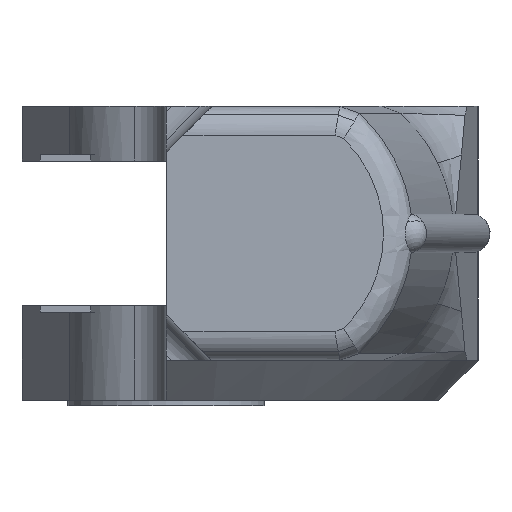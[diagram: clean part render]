
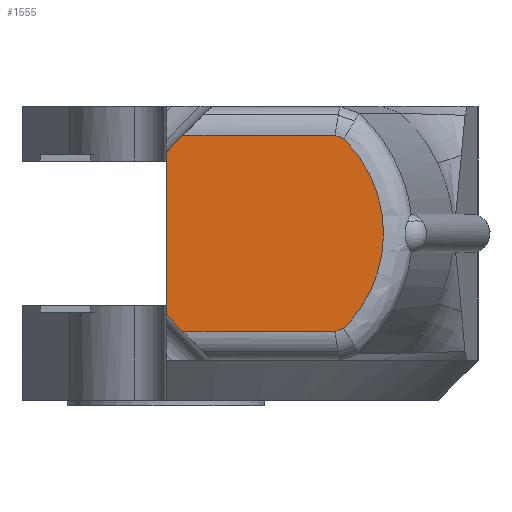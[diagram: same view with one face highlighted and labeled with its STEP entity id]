
A CAD part, left-side view. The second image highlights one B-rep face of the part: STEP entity #1555.
In plain terms, the highlighted planar face has unit normal (-1, 0, 0).
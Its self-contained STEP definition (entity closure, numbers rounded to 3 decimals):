
#22 = CARTESIAN_POINT ( 'NONE',  ( -27.856, 0., -2.85 ) ) ;
#83 = ORIENTED_EDGE ( 'NONE', *, *, #1610, .F. ) ;
#96 = DIRECTION ( 'NONE',  ( -1., 0., 0. ) ) ;
#164 = VECTOR ( 'NONE', #2389, 1000. ) ;
#197 = ORIENTED_EDGE ( 'NONE', *, *, #1725, .F. ) ;
#244 = VECTOR ( 'NONE', #807, 1000. ) ;
#266 = CARTESIAN_POINT ( 'NONE',  ( -27.856, -0.091, 2.941 ) ) ;
#279 = CARTESIAN_POINT ( 'NONE',  ( -27.856, 0., 0. ) ) ;
#336 = VECTOR ( 'NONE', #1314, 1000. ) ;
#350 = DIRECTION ( 'NONE',  ( 0., 1., 0. ) ) ;
#390 = DIRECTION ( 'NONE',  ( 0., -0.939, -0.343 ) ) ;
#400 = VERTEX_POINT ( 'NONE', #1498 ) ;
#481 = CARTESIAN_POINT ( 'NONE',  ( -27.856, 0., 2.85 ) ) ;
#652 = CARTESIAN_POINT ( 'NONE',  ( -27.856, -3.89, 4.185 ) ) ;
#695 = CARTESIAN_POINT ( 'NONE',  ( -27.856, -6.233, 3.329 ) ) ;
#807 = DIRECTION ( 'NONE',  ( 0., 0.707, -0.707 ) ) ;
#813 = VECTOR ( 'NONE', #350, 1000. ) ;
#892 = CARTESIAN_POINT ( 'NONE',  ( -27.856, -2.016, 3.442 ) ) ;
#923 = VECTOR ( 'NONE', #1765, 1000. ) ;
#926 = CARTESIAN_POINT ( 'NONE',  ( -27.856, -0.591, -3.442 ) ) ;
#934 = VERTEX_POINT ( 'NONE', #22 ) ;
#944 = LINE ( 'NONE', #279, #164 ) ;
#1031 = LINE ( 'NONE', #1042, #336 ) ;
#1038 = VERTEX_POINT ( 'NONE', #1669 ) ;
#1042 = CARTESIAN_POINT ( 'NONE',  ( -27.856, 0.713, -2.138 ) ) ;
#1099 = CARTESIAN_POINT ( 'NONE',  ( -27.856, -5.925, 3.442 ) ) ;
#1104 = VERTEX_POINT ( 'NONE', #1716 ) ;
#1221 = CARTESIAN_POINT ( 'NONE',  ( -27.856, -8.217, -1.386 ) ) ;
#1314 = DIRECTION ( 'NONE',  ( 0., -0.707, -0.707 ) ) ;
#1444 = EDGE_LOOP ( 'NONE', ( #3081, #197, #3039, #83, #2172, #3075, #2840, #2040 ) ) ;
#1498 = CARTESIAN_POINT ( 'NONE',  ( -27.856, -0.591, 3.442 ) ) ;
#1535 = EDGE_CURVE ( 'NONE', #1038, #1642, #2214, .T. ) ;
#1555 = ADVANCED_FACE ( 'NONE', ( #2903 ), #2462, .T. ) ;
#1578 = EDGE_CURVE ( 'NONE', #400, #2092, #2044, .T. ) ;
#1610 = EDGE_CURVE ( 'NONE', #2092, #3368, #1970, .T. ) ;
#1642 = VERTEX_POINT ( 'NONE', #926 ) ;
#1660 = LINE ( 'NONE', #266, #244 ) ;
#1669 = CARTESIAN_POINT ( 'NONE',  ( -27.856, -5.925, -3.442 ) ) ;
#1682 = EDGE_CURVE ( 'NONE', #3368, #1104, #2667, .T. ) ;
#1716 = CARTESIAN_POINT ( 'NONE',  ( -27.856, -6.233, -3.329 ) ) ;
#1725 = EDGE_CURVE ( 'NONE', #1104, #1038, #2324, .T. ) ;
#1765 = DIRECTION ( 'NONE',  ( 0., 0.939, -0.343 ) ) ;
#1874 = VERTEX_POINT ( 'NONE', #481 ) ;
#1928 = CARTESIAN_POINT ( 'NONE',  ( -27.856, -6.233, 3.329 ) ) ;
#1930 = CARTESIAN_POINT ( 'NONE',  ( -27.856, -2.016, -3.442 ) ) ;
#1944 = CARTESIAN_POINT ( 'NONE',  ( -27.856, 0., 0. ) ) ;
#1966 = DIRECTION ( 'NONE',  ( 0., -1., 0. ) ) ;
#1970 = LINE ( 'NONE', #652, #2572 ) ;
#1972 = EDGE_CURVE ( 'NONE', #934, #1642, #1031, .T. ) ;
#1990 = AXIS2_PLACEMENT_3D ( 'NONE', #1944, #96, #2739 ) ;
#2008 = CARTESIAN_POINT ( 'NONE',  ( -27.856, -8.217, 1.386 ) ) ;
#2011 = EDGE_CURVE ( 'NONE', #400, #1874, #1660, .T. ) ;
#2029 = EDGE_CURVE ( 'NONE', #1874, #934, #944, .T. ) ;
#2040 = ORIENTED_EDGE ( 'NONE', *, *, #1972, .T. ) ;
#2044 = LINE ( 'NONE', #892, #3326 ) ;
#2092 = VERTEX_POINT ( 'NONE', #1099 ) ;
#2172 = ORIENTED_EDGE ( 'NONE', *, *, #1578, .F. ) ;
#2214 = LINE ( 'NONE', #1930, #813 ) ;
#2324 = LINE ( 'NONE', #3055, #923 ) ;
#2389 = DIRECTION ( 'NONE',  ( 0., 0., -1. ) ) ;
#2462 = PLANE ( 'NONE',  #1990 ) ;
#2572 = VECTOR ( 'NONE', #390, 1000. ) ;
#2667 =( BOUNDED_CURVE ( )  B_SPLINE_CURVE ( 3, ( #695, #2008, #1221, #3047 ),
 .UNSPECIFIED., .F., .F. ) 
 B_SPLINE_CURVE_WITH_KNOTS ( ( 4, 4 ),
 ( 5.489, 7.077 ),
 .UNSPECIFIED. ) 
 CURVE ( )  GEOMETRIC_REPRESENTATION_ITEM ( )  RATIONAL_B_SPLINE_CURVE ( ( 1., 0.801, 0.801, 1. ) ) 
 REPRESENTATION_ITEM ( '' )  );
#2739 = DIRECTION ( 'NONE',  ( 0., -1., 0. ) ) ;
#2840 = ORIENTED_EDGE ( 'NONE', *, *, #2029, .T. ) ;
#2903 = FACE_OUTER_BOUND ( 'NONE', #1444, .T. ) ;
#3039 = ORIENTED_EDGE ( 'NONE', *, *, #1682, .F. ) ;
#3047 = CARTESIAN_POINT ( 'NONE',  ( -27.856, -6.233, -3.329 ) ) ;
#3055 = CARTESIAN_POINT ( 'NONE',  ( -27.856, -3.89, -4.185 ) ) ;
#3075 = ORIENTED_EDGE ( 'NONE', *, *, #2011, .T. ) ;
#3081 = ORIENTED_EDGE ( 'NONE', *, *, #1535, .F. ) ;
#3326 = VECTOR ( 'NONE', #1966, 1000. ) ;
#3368 = VERTEX_POINT ( 'NONE', #1928 ) ;
